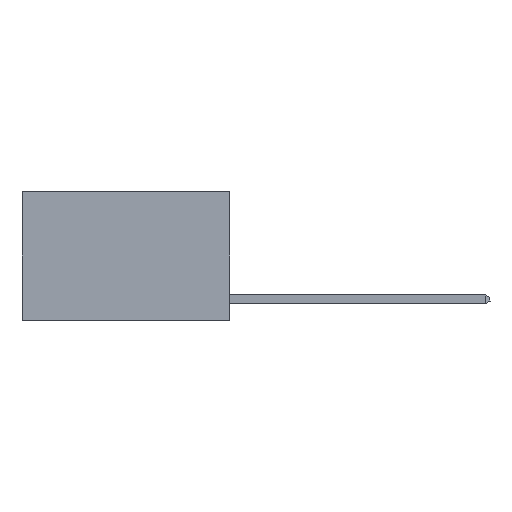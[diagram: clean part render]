
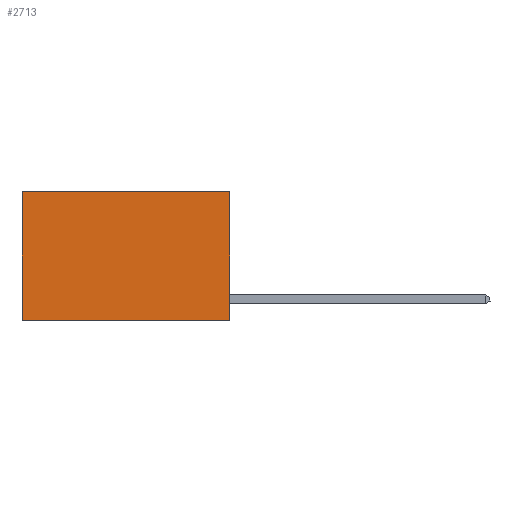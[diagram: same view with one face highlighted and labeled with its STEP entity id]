
A CAD part, left-side view. The second image highlights one B-rep face of the part: STEP entity #2713.
In plain terms, the highlighted planar face has unit normal (-1, 0, 0).
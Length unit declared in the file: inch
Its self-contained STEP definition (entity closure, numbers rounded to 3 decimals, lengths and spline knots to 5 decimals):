
#330 = VECTOR ( 'NONE', #6723, 39.37008 ) ;
#553 = DIRECTION ( 'NONE',  ( 0., 0., -1. ) ) ;
#722 = DIRECTION ( 'NONE',  ( 0., 1., 0. ) ) ;
#813 = VERTEX_POINT ( 'NONE', #9364 ) ;
#1033 = CARTESIAN_POINT ( 'NONE',  ( 0.2625, 0., 0. ) ) ;
#1034 = CARTESIAN_POINT ( 'NONE',  ( 0.2625, 0.6, -0.37 ) ) ;
#1306 = EDGE_LOOP ( 'NONE', ( #5102, #6503, #5564, #4474 ) ) ;
#1511 = CARTESIAN_POINT ( 'NONE',  ( 0.2625, 0., 0. ) ) ;
#2512 = FACE_OUTER_BOUND ( 'NONE', #1306, .T. ) ;
#2520 = CARTESIAN_POINT ( 'NONE',  ( 0.2625, 0.6, 0. ) ) ;
#2713 = ADVANCED_FACE ( 'NONE', ( #2512 ), #2732, .F. ) ;
#2732 = PLANE ( 'NONE',  #8021 ) ;
#3156 = EDGE_CURVE ( 'NONE', #5489, #813, #6870, .T. ) ;
#4113 = CARTESIAN_POINT ( 'NONE',  ( 0.2625, 0., 0. ) ) ;
#4474 = ORIENTED_EDGE ( 'NONE', *, *, #9088, .T. ) ;
#4570 = LINE ( 'NONE', #6695, #330 ) ;
#4636 = EDGE_CURVE ( 'NONE', #5634, #7317, #7336, .T. ) ;
#4808 = DIRECTION ( 'NONE',  ( 0., 0., -1. ) ) ;
#4867 = DIRECTION ( 'NONE',  ( 0., 0., -1. ) ) ;
#5102 = ORIENTED_EDGE ( 'NONE', *, *, #4636, .T. ) ;
#5489 = VERTEX_POINT ( 'NONE', #1511 ) ;
#5564 = ORIENTED_EDGE ( 'NONE', *, *, #3156, .F. ) ;
#5577 = VECTOR ( 'NONE', #722, 39.37008 ) ;
#5591 = CARTESIAN_POINT ( 'NONE',  ( 0.2625, 0.6, 0. ) ) ;
#5634 = VERTEX_POINT ( 'NONE', #5591 ) ;
#6372 = EDGE_CURVE ( 'NONE', #813, #7317, #4570, .T. ) ;
#6503 = ORIENTED_EDGE ( 'NONE', *, *, #6372, .F. ) ;
#6695 = CARTESIAN_POINT ( 'NONE',  ( 0.2625, 0., -0.37 ) ) ;
#6723 = DIRECTION ( 'NONE',  ( 0., 1., 0. ) ) ;
#6870 = LINE ( 'NONE', #4113, #9233 ) ;
#7317 = VERTEX_POINT ( 'NONE', #1034 ) ;
#7336 = LINE ( 'NONE', #2520, #9562 ) ;
#8021 = AXIS2_PLACEMENT_3D ( 'NONE', #1033, #8837, #553 ) ;
#8837 = DIRECTION ( 'NONE',  ( 1., 0., 0. ) ) ;
#9088 = EDGE_CURVE ( 'NONE', #5489, #5634, #9596, .T. ) ;
#9233 = VECTOR ( 'NONE', #4867, 39.37008 ) ;
#9364 = CARTESIAN_POINT ( 'NONE',  ( 0.2625, 0., -0.37 ) ) ;
#9562 = VECTOR ( 'NONE', #4808, 39.37008 ) ;
#9596 = LINE ( 'NONE', #9752, #5577 ) ;
#9752 = CARTESIAN_POINT ( 'NONE',  ( 0.2625, 0., 0. ) ) ;
